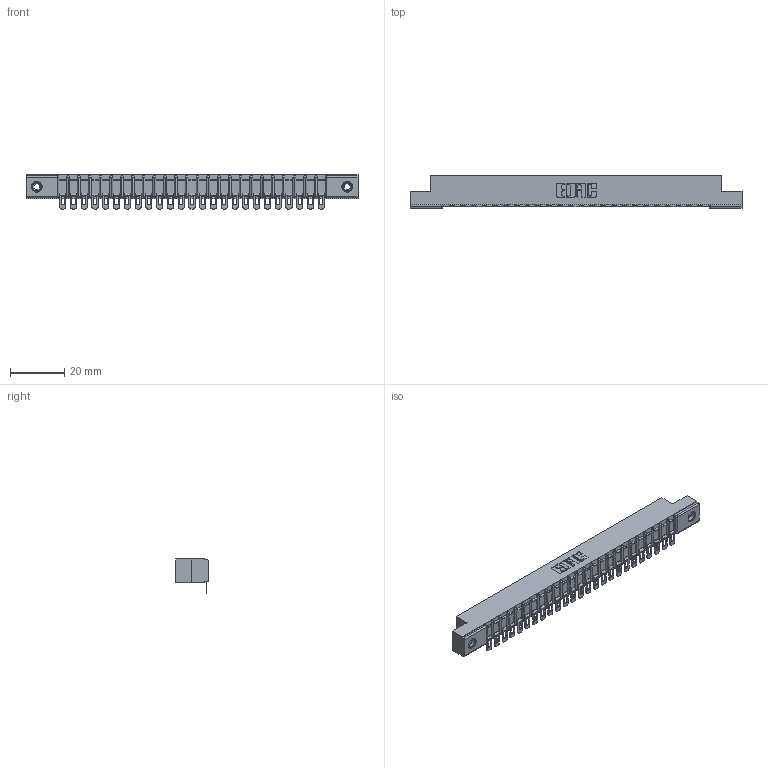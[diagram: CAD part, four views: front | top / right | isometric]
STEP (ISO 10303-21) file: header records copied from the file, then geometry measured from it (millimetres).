
FILE_DESCRIPTION (( 'STEP AP203' ), '1' );
FILE_NAME ('357-025-554-108.STEP', '2019-09-17T00:48:03', ( '' ), ( '' ), 'SwSTEP 2.0', 'SolidWorks 2016', '' );
FILE_SCHEMA (( 'CONFIG_CONTROL_DESIGN' ));
Length unit declared in the file: inch
Products named in the file (4): 357-025-554-108; 307 Part_.156 Dia Mounting Holes; 345-250-001_345-250-003-102; 307-290-002_554
Assembly tree (28 placements, depth 2):
  357-025-554-108
    307 Part_.156 Dia Mounting Holes
    307-290-002_554  x25
    345-250-001_345-250-003-102  x2
Bounding box: 122.07 x 12.01 x 12.52 mm (x, y, z)
Volume: 8063 mm3; surface area: 14953.7 mm2
Topology: 28 solids, 28 shells, 2229 faces, 6784 edges, 4444 vertices
Faces by surface type: plane 1252, cylinder 909, sphere 52, cone 12, torus 4
Entity records: 25678 total; most frequent: CARTESIAN_POINT 4309, ORIENTED_EDGE 4292, DIRECTION 4210, EDGE_CURVE 2146, VECTOR 1628, LINE 1628, VERTEX_POINT 1390, AXIS2_PLACEMENT_3D 1291
